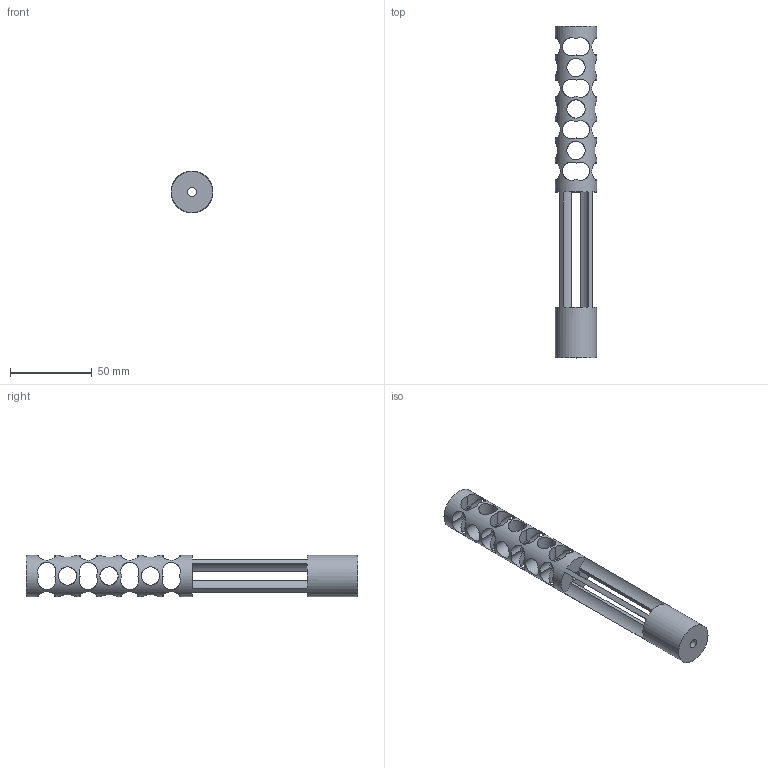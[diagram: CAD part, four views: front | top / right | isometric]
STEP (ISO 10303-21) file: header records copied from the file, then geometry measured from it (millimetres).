
FILE_DESCRIPTION(/* description */ (''),/* implementation_level */ '2;1');
FILE_NAME(/* name */ 'Monocore desgin.stp',/* time_stamp */ '2015-05-04T13:35:52-05:00',/* author */ ('Matt'),/* organization */ (''),/* preprocessor_version */ 'ST-DEVELOPER v15.6',/* originating_system */ 'Autodesk Inventor 2015',/* authorisation */ '');
FILE_SCHEMA (('AUTOMOTIVE_DESIGN { 1 0 10303 214 3 1 1 }'));
Length unit declared in the file: inch
Products named in the file (1): Monocore desgin
Bounding box: 25.4 x 203.2 x 25.4 mm (x, y, z)
Volume: 37478 mm3; surface area: 23446.8 mm2
Topology: 1 solids, 1 shells, 106 faces, 381 edges, 239 vertices
Faces by surface type: cylinder 94, plane 12
Full cylindrical faces by diameter (mm): 5.588 x9, 11.176 x12, 25.4 x1
Entity records: 5482 total; most frequent: CARTESIAN_POINT 2435, ORIENTED_EDGE 668, DIRECTION 590, EDGE_CURVE 334, AXIS2_PLACEMENT_3D 261, VERTEX_POINT 222, EDGE_LOOP 164, ELLIPSE 124
